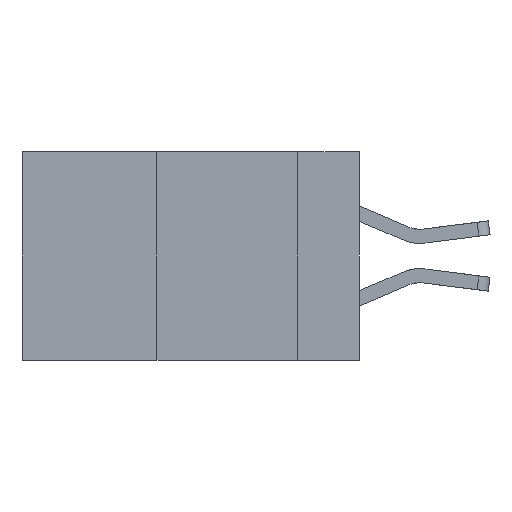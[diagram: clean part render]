
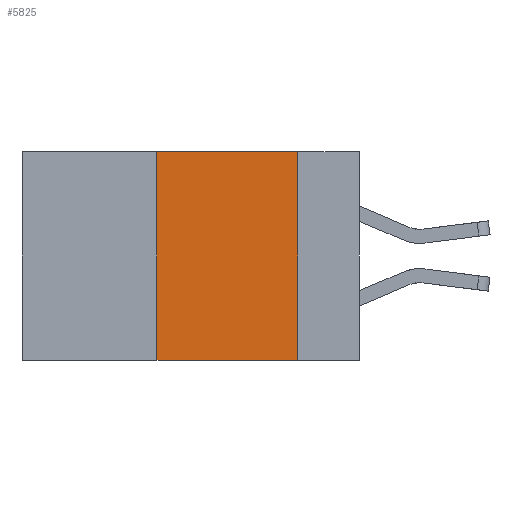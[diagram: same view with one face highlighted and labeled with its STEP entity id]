
A CAD part, left-side view. The second image highlights one B-rep face of the part: STEP entity #5825.
In plain terms, the highlighted planar face has unit normal (-1, 0, 0).
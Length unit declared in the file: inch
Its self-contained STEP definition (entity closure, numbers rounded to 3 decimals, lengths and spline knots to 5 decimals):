
#449 = VECTOR ( 'NONE', #1842, 39.37008 ) ;
#755 = CARTESIAN_POINT ( 'NONE',  ( 0., 0.6, 0. ) ) ;
#834 = VERTEX_POINT ( 'NONE', #1751 ) ;
#1349 = VECTOR ( 'NONE', #9280, 39.37008 ) ;
#1751 = CARTESIAN_POINT ( 'NONE',  ( 0., 0.36, -0.37 ) ) ;
#1759 = LINE ( 'NONE', #7326, #7526 ) ;
#1842 = DIRECTION ( 'NONE',  ( 0., -1., 0. ) ) ;
#2319 = DIRECTION ( 'NONE',  ( 0., 0., -1. ) ) ;
#2479 = VERTEX_POINT ( 'NONE', #13048 ) ;
#2488 = ORIENTED_EDGE ( 'NONE', *, *, #3823, .T. ) ;
#2614 = CARTESIAN_POINT ( 'NONE',  ( 0., 0.36, 0. ) ) ;
#3823 = EDGE_CURVE ( 'NONE', #834, #11279, #8605, .T. ) ;
#3850 = ORIENTED_EDGE ( 'NONE', *, *, #11265, .F. ) ;
#4843 = LINE ( 'NONE', #2614, #1349 ) ;
#4869 = ORIENTED_EDGE ( 'NONE', *, *, #6953, .F. ) ;
#5568 = FACE_OUTER_BOUND ( 'NONE', #12521, .T. ) ;
#5825 = ADVANCED_FACE ( 'NONE', ( #5568 ), #6662, .F. ) ;
#6208 = VERTEX_POINT ( 'NONE', #9764 ) ;
#6662 = PLANE ( 'NONE',  #10571 ) ;
#6714 = CARTESIAN_POINT ( 'NONE',  ( 0., 0.6, -0.37 ) ) ;
#6953 = EDGE_CURVE ( 'NONE', #2479, #11279, #1759, .T. ) ;
#7326 = CARTESIAN_POINT ( 'NONE',  ( 0., 0.11, 0. ) ) ;
#7526 = VECTOR ( 'NONE', #8557, 39.37008 ) ;
#7873 = DIRECTION ( 'NONE',  ( 0., -1., 0. ) ) ;
#8557 = DIRECTION ( 'NONE',  ( 0., 0., -1. ) ) ;
#8605 = LINE ( 'NONE', #6714, #13548 ) ;
#8903 = ORIENTED_EDGE ( 'NONE', *, *, #10122, .F. ) ;
#9280 = DIRECTION ( 'NONE',  ( 0., 0., 1. ) ) ;
#9764 = CARTESIAN_POINT ( 'NONE',  ( 0., 0.36, 0. ) ) ;
#10077 = DIRECTION ( 'NONE',  ( 1., 0., 0. ) ) ;
#10122 = EDGE_CURVE ( 'NONE', #834, #6208, #4843, .T. ) ;
#10571 = AXIS2_PLACEMENT_3D ( 'NONE', #11099, #10077, #2319 ) ;
#10696 = CARTESIAN_POINT ( 'NONE',  ( 0., 0.11, -0.37 ) ) ;
#10830 = LINE ( 'NONE', #755, #449 ) ;
#11099 = CARTESIAN_POINT ( 'NONE',  ( 0., 0.6, 0. ) ) ;
#11265 = EDGE_CURVE ( 'NONE', #6208, #2479, #10830, .T. ) ;
#11279 = VERTEX_POINT ( 'NONE', #10696 ) ;
#12521 = EDGE_LOOP ( 'NONE', ( #4869, #3850, #8903, #2488 ) ) ;
#13048 = CARTESIAN_POINT ( 'NONE',  ( 0., 0.11, 0. ) ) ;
#13548 = VECTOR ( 'NONE', #7873, 39.37008 ) ;
